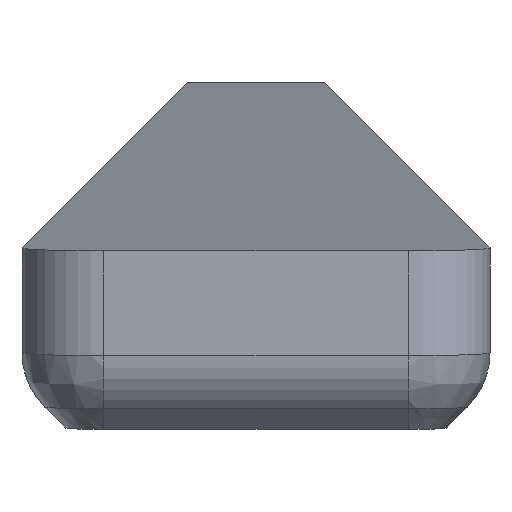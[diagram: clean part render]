
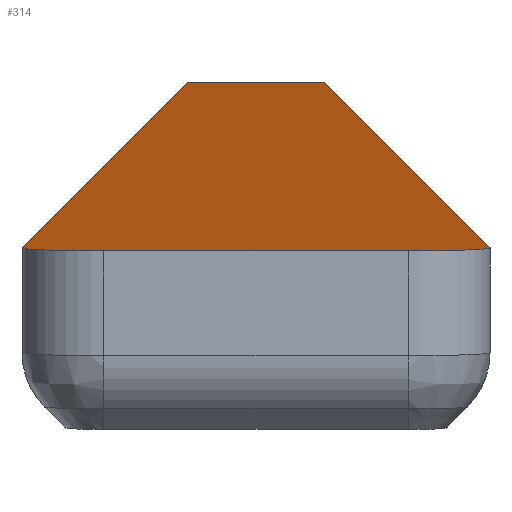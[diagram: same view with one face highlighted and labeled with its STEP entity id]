
A CAD part, front view. The second image highlights one B-rep face of the part: STEP entity #314.
In plain terms, the highlighted planar face has unit normal (0, -0.035, 0.999).
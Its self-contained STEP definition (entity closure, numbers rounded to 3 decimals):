
#27=CIRCLE('',#346,0.75);
#28=CIRCLE('',#350,0.75);
#40=PLANE('',#360);
#60=FACE_OUTER_BOUND('',#80,.T.);
#80=EDGE_LOOP('',(#283,#284,#285,#286,#287,#288));
#84=LINE('',#469,#112);
#93=LINE('',#529,#121);
#96=LINE('',#537,#124);
#101=LINE('',#549,#129);
#112=VECTOR('',#374,10.);
#121=VECTOR('',#407,10.);
#124=VECTOR('',#416,10.);
#129=VECTOR('',#429,10.);
#143=VERTEX_POINT('',#466);
#144=VERTEX_POINT('',#468);
#153=VERTEX_POINT('',#527);
#154=VERTEX_POINT('',#531);
#155=VERTEX_POINT('',#535);
#158=VERTEX_POINT('',#545);
#168=EDGE_CURVE('',#144,#143,#84,.T.);
#185=EDGE_CURVE('',#143,#153,#93,.T.);
#187=EDGE_CURVE('',#154,#153,#27,.F.);
#189=EDGE_CURVE('',#154,#155,#96,.T.);
#194=EDGE_CURVE('',#158,#155,#28,.F.);
#195=EDGE_CURVE('',#158,#144,#101,.T.);
#283=ORIENTED_EDGE('',*,*,#187,.F.);
#284=ORIENTED_EDGE('',*,*,#189,.T.);
#285=ORIENTED_EDGE('',*,*,#194,.F.);
#286=ORIENTED_EDGE('',*,*,#195,.T.);
#287=ORIENTED_EDGE('',*,*,#168,.T.);
#288=ORIENTED_EDGE('',*,*,#185,.T.);
#314=ADVANCED_FACE('',(#60),#40,.T.);
#346=AXIS2_PLACEMENT_3D('',#533,#411,#412);
#350=AXIS2_PLACEMENT_3D('',#547,#425,#426);
#360=AXIS2_PLACEMENT_3D('',#569,#453,#454);
#374=DIRECTION('',(-1.,0.,0.));
#407=DIRECTION('',(-0.035,-0.999,-0.035));
#411=DIRECTION('center_axis',(0.,-0.035,0.999));
#412=DIRECTION('ref_axis',(-0.719,-0.694,-0.024));
#416=DIRECTION('',(1.,0.,0.));
#425=DIRECTION('center_axis',(0.,-0.035,0.999));
#426=DIRECTION('ref_axis',(0.719,-0.694,-0.024));
#429=DIRECTION('',(-0.035,0.999,0.035));
#453=DIRECTION('center_axis',(0.,-0.035,0.999));
#454=DIRECTION('ref_axis',(1.,0.,0.));
#466=CARTESIAN_POINT('',(-0.629,52.791,5.921));
#468=CARTESIAN_POINT('',(0.629,52.791,5.921));
#469=CARTESIAN_POINT('',(0.302,52.791,5.921));
#527=CARTESIAN_POINT('',(-2.143,9.457,4.407));
#529=CARTESIAN_POINT('',(-0.926,44.309,5.625));
#531=CARTESIAN_POINT('',(-1.393,8.681,4.38));
#533=CARTESIAN_POINT('Origin',(-1.393,9.431,4.407));
#535=CARTESIAN_POINT('',(1.393,8.681,4.38));
#537=CARTESIAN_POINT('',(-0.557,8.681,4.38));
#545=CARTESIAN_POINT('',(2.143,9.457,4.407));
#547=CARTESIAN_POINT('Origin',(1.393,9.431,4.407));
#549=CARTESIAN_POINT('',(1.555,26.289,4.995));
#569=CARTESIAN_POINT('Origin',(0.,35.083,5.302));
